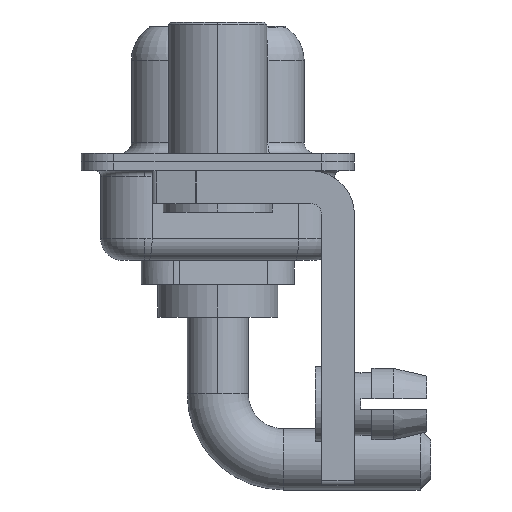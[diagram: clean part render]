
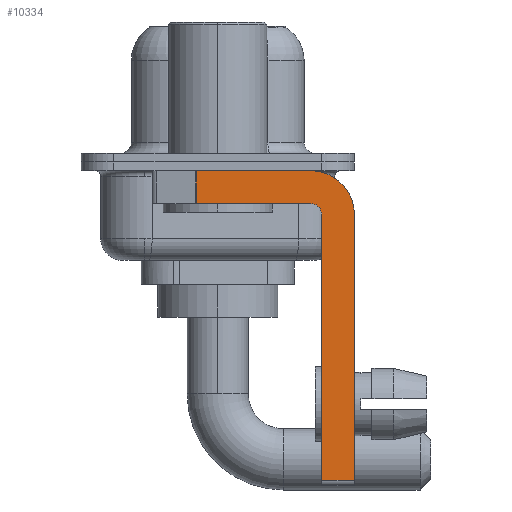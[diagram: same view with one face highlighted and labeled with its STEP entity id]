
A CAD part, left-side view. The second image highlights one B-rep face of the part: STEP entity #10334.
In plain terms, the highlighted planar face has unit normal (-1, 0, 0).
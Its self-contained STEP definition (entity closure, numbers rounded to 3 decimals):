
#148 = VERTEX_POINT ( 'NONE', #15916 ) ;
#156 = VECTOR ( 'NONE', #11842, 1000. ) ;
#438 = VECTOR ( 'NONE', #16236, 1000. ) ;
#504 = CARTESIAN_POINT ( 'NONE',  ( -2.9, -4.25, -1.9 ) ) ;
#661 = AXIS2_PLACEMENT_3D ( 'NONE', #9208, #8290, #10694 ) ;
#708 = DIRECTION ( 'NONE',  ( 0., -1., 0. ) ) ;
#896 = CARTESIAN_POINT ( 'NONE',  ( -2.9, -6.25, -2.4 ) ) ;
#1150 = DIRECTION ( 'NONE',  ( 0., 0., -1. ) ) ;
#1170 = CARTESIAN_POINT ( 'NONE',  ( -2.9, -4.25, -2.4 ) ) ;
#1931 = LINE ( 'NONE', #9444, #156 ) ;
#2102 = VERTEX_POINT ( 'NONE', #9715 ) ;
#2444 = ORIENTED_EDGE ( 'NONE', *, *, #8073, .F. ) ;
#2554 = VECTOR ( 'NONE', #9887, 1000. ) ;
#2688 = EDGE_CURVE ( 'NONE', #14629, #148, #1931, .T. ) ;
#3452 = CARTESIAN_POINT ( 'NONE',  ( -2.9, 0.978, -1.9 ) ) ;
#3509 = AXIS2_PLACEMENT_3D ( 'NONE', #12978, #5312, #7765 ) ;
#3651 = VERTEX_POINT ( 'NONE', #4586 ) ;
#3720 = PLANE ( 'NONE',  #8729 ) ;
#3792 = DIRECTION ( 'NONE',  ( 0., 0., -1. ) ) ;
#4586 = CARTESIAN_POINT ( 'NONE',  ( -2.9, -6.25, -14.55 ) ) ;
#4966 = FACE_OUTER_BOUND ( 'NONE', #10564, .T. ) ;
#5312 = DIRECTION ( 'NONE',  ( 1., 0., 0. ) ) ;
#5700 = EDGE_CURVE ( 'NONE', #14629, #11164, #14838, .T. ) ;
#5756 = ORIENTED_EDGE ( 'NONE', *, *, #5700, .T. ) ;
#5819 = EDGE_CURVE ( 'NONE', #6545, #11164, #11214, .T. ) ;
#6233 = EDGE_CURVE ( 'NONE', #13459, #3651, #6286, .T. ) ;
#6286 = LINE ( 'NONE', #10098, #8096 ) ;
#6425 = ORIENTED_EDGE ( 'NONE', *, *, #5819, .F. ) ;
#6545 = VERTEX_POINT ( 'NONE', #504 ) ;
#6962 = ORIENTED_EDGE ( 'NONE', *, *, #2688, .F. ) ;
#7183 = CIRCLE ( 'NONE', #3509, 2. ) ;
#7765 = DIRECTION ( 'NONE',  ( 0., 0., -1. ) ) ;
#8037 = ORIENTED_EDGE ( 'NONE', *, *, #14677, .F. ) ;
#8073 = EDGE_CURVE ( 'NONE', #148, #10276, #7183, .T. ) ;
#8096 = VECTOR ( 'NONE', #708, 1000. ) ;
#8290 = DIRECTION ( 'NONE',  ( -1., 0., 0. ) ) ;
#8425 = VECTOR ( 'NONE', #16266, 1000. ) ;
#8729 = AXIS2_PLACEMENT_3D ( 'NONE', #1170, #11153, #3792 ) ;
#9208 = CARTESIAN_POINT ( 'NONE',  ( -2.9, -4.25, -2.4 ) ) ;
#9444 = CARTESIAN_POINT ( 'NONE',  ( -2.9, 3., -0.4 ) ) ;
#9481 = EDGE_CURVE ( 'NONE', #10276, #3651, #11051, .T. ) ;
#9715 = CARTESIAN_POINT ( 'NONE',  ( -2.9, -4.75, -2.4 ) ) ;
#9742 = EDGE_CURVE ( 'NONE', #2102, #6545, #11466, .T. ) ;
#9887 = DIRECTION ( 'NONE',  ( 0., 0., -1. ) ) ;
#10098 = CARTESIAN_POINT ( 'NONE',  ( -2.9, -4.25, -14.55 ) ) ;
#10161 = LINE ( 'NONE', #11245, #8425 ) ;
#10276 = VERTEX_POINT ( 'NONE', #14528 ) ;
#10285 = CARTESIAN_POINT ( 'NONE',  ( -2.9, -4.25, -1.9 ) ) ;
#10334 = ADVANCED_FACE ( 'NONE', ( #4966 ), #3720, .F. ) ;
#10564 = EDGE_LOOP ( 'NONE', ( #6962, #5756, #6425, #12425, #8037, #16129, #11025, #2444 ) ) ;
#10694 = DIRECTION ( 'NONE',  ( 0., 0., 1. ) ) ;
#11025 = ORIENTED_EDGE ( 'NONE', *, *, #9481, .F. ) ;
#11051 = LINE ( 'NONE', #896, #12739 ) ;
#11153 = DIRECTION ( 'NONE',  ( 1., 0., 0. ) ) ;
#11164 = VERTEX_POINT ( 'NONE', #14495 ) ;
#11214 = LINE ( 'NONE', #10285, #438 ) ;
#11245 = CARTESIAN_POINT ( 'NONE',  ( -2.9, -4.75, -14.8 ) ) ;
#11466 = CIRCLE ( 'NONE', #661, 0.5 ) ;
#11557 = CARTESIAN_POINT ( 'NONE',  ( -2.9, -4.75, -14.55 ) ) ;
#11842 = DIRECTION ( 'NONE',  ( 0., -1., 0. ) ) ;
#12425 = ORIENTED_EDGE ( 'NONE', *, *, #9742, .F. ) ;
#12739 = VECTOR ( 'NONE', #1150, 1000. ) ;
#12978 = CARTESIAN_POINT ( 'NONE',  ( -2.9, -4.25, -2.4 ) ) ;
#13459 = VERTEX_POINT ( 'NONE', #11557 ) ;
#14495 = CARTESIAN_POINT ( 'NONE',  ( -2.9, 0.978, -1.9 ) ) ;
#14528 = CARTESIAN_POINT ( 'NONE',  ( -2.9, -6.25, -2.4 ) ) ;
#14629 = VERTEX_POINT ( 'NONE', #15191 ) ;
#14677 = EDGE_CURVE ( 'NONE', #13459, #2102, #10161, .T. ) ;
#14838 = LINE ( 'NONE', #3452, #2554 ) ;
#15191 = CARTESIAN_POINT ( 'NONE',  ( -2.9, 0.978, -0.4 ) ) ;
#15916 = CARTESIAN_POINT ( 'NONE',  ( -2.9, -4.25, -0.4 ) ) ;
#16129 = ORIENTED_EDGE ( 'NONE', *, *, #6233, .T. ) ;
#16236 = DIRECTION ( 'NONE',  ( 0., 1., 0. ) ) ;
#16266 = DIRECTION ( 'NONE',  ( 0., 0., 1. ) ) ;
